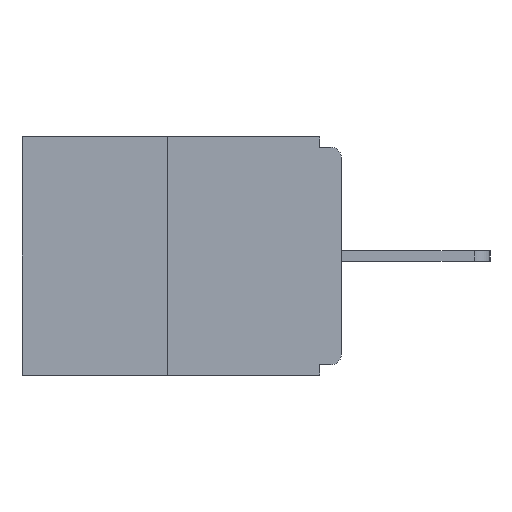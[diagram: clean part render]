
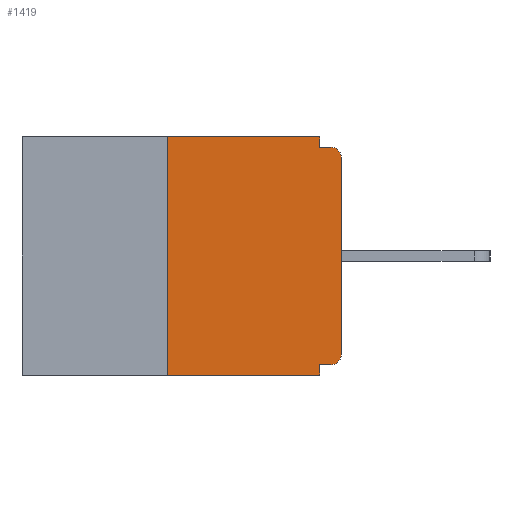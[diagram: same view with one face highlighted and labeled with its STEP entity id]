
A CAD part, left-side view. The second image highlights one B-rep face of the part: STEP entity #1419.
In plain terms, the highlighted planar face has unit normal (-1, 0, 0).
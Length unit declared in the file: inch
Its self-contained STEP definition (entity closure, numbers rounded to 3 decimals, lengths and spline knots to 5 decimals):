
#218 = VERTEX_POINT ( 'NONE', #4990 ) ;
#247 = VERTEX_POINT ( 'NONE', #21873 ) ;
#273 = LINE ( 'NONE', #2394, #9201 ) ;
#301 = CIRCLE ( 'NONE', #13572, 0.015 ) ;
#479 = LINE ( 'NONE', #7695, #22213 ) ;
#814 = DIRECTION ( 'NONE',  ( 0., 0., 1. ) ) ;
#1419 = ADVANCED_FACE ( 'NONE', ( #20451 ), #12638, .F. ) ;
#1489 = DIRECTION ( 'NONE',  ( 1., 0., 0. ) ) ;
#1607 = VECTOR ( 'NONE', #2393, 39.37008 ) ;
#1997 = CARTESIAN_POINT ( 'NONE',  ( 0., 0.031, -0.343 ) ) ;
#2081 = VECTOR ( 'NONE', #15148, 39.37008 ) ;
#2185 = LINE ( 'NONE', #17173, #2081 ) ;
#2393 = DIRECTION ( 'NONE',  ( 0., 0., -1. ) ) ;
#2394 = CARTESIAN_POINT ( 'NONE',  ( 0., 0., -0.015 ) ) ;
#2849 = EDGE_CURVE ( 'NONE', #15217, #17095, #2185, .T. ) ;
#3319 = EDGE_CURVE ( 'NONE', #11596, #247, #479, .T. ) ;
#4198 = ORIENTED_EDGE ( 'NONE', *, *, #2849, .F. ) ;
#4282 = LINE ( 'NONE', #9743, #1607 ) ;
#4823 = ORIENTED_EDGE ( 'NONE', *, *, #10709, .F. ) ;
#4830 = DIRECTION ( 'NONE',  ( 0., 0., -1. ) ) ;
#4950 = ORIENTED_EDGE ( 'NONE', *, *, #3319, .T. ) ;
#4990 = CARTESIAN_POINT ( 'NONE',  ( 0., 0.031, 0. ) ) ;
#5284 = EDGE_CURVE ( 'NONE', #11596, #22111, #11060, .T. ) ;
#5548 = LINE ( 'NONE', #1997, #19799 ) ;
#5707 = DIRECTION ( 'NONE',  ( 0., 0., 1. ) ) ;
#6445 = DIRECTION ( 'NONE',  ( 0., -1., 0. ) ) ;
#7033 = CARTESIAN_POINT ( 'NONE',  ( 0., 0.46, 0. ) ) ;
#7054 = ORIENTED_EDGE ( 'NONE', *, *, #21205, .F. ) ;
#7293 = CARTESIAN_POINT ( 'NONE',  ( 0., 0.015, -0.313 ) ) ;
#7461 = ORIENTED_EDGE ( 'NONE', *, *, #16400, .T. ) ;
#7664 = DIRECTION ( 'NONE',  ( 0., 0., -1. ) ) ;
#7695 = CARTESIAN_POINT ( 'NONE',  ( 0., 0.46, -0.343 ) ) ;
#9201 = VECTOR ( 'NONE', #16448, 39.37008 ) ;
#9293 = VECTOR ( 'NONE', #814, 39.37008 ) ;
#9549 = DIRECTION ( 'NONE',  ( -1., 0., 0. ) ) ;
#9743 = CARTESIAN_POINT ( 'NONE',  ( 0., 0.031, 0. ) ) ;
#9763 = VERTEX_POINT ( 'NONE', #18137 ) ;
#9778 = CARTESIAN_POINT ( 'NONE',  ( 0., 0., -0.313 ) ) ;
#10496 = VECTOR ( 'NONE', #5707, 39.37008 ) ;
#10709 = EDGE_CURVE ( 'NONE', #17095, #247, #5548, .T. ) ;
#11039 = CARTESIAN_POINT ( 'NONE',  ( 0., 0.031, -0.328 ) ) ;
#11060 = LINE ( 'NONE', #11299, #10496 ) ;
#11299 = CARTESIAN_POINT ( 'NONE',  ( 0., 0.25, 0. ) ) ;
#11584 = EDGE_CURVE ( 'NONE', #22111, #218, #15273, .T. ) ;
#11596 = VERTEX_POINT ( 'NONE', #22624 ) ;
#11966 = ORIENTED_EDGE ( 'NONE', *, *, #12019, .F. ) ;
#11976 = ORIENTED_EDGE ( 'NONE', *, *, #5284, .F. ) ;
#12019 = EDGE_CURVE ( 'NONE', #218, #16827, #4282, .T. ) ;
#12638 = PLANE ( 'NONE',  #12646 ) ;
#12646 = AXIS2_PLACEMENT_3D ( 'NONE', #7033, #1489, #14985 ) ;
#13403 = LINE ( 'NONE', #17122, #9293 ) ;
#13423 = CARTESIAN_POINT ( 'NONE',  ( 0., 0.031, -0.015 ) ) ;
#13515 = DIRECTION ( 'NONE',  ( -1., 0., 0. ) ) ;
#13572 = AXIS2_PLACEMENT_3D ( 'NONE', #18893, #13515, #4830 ) ;
#14664 = VERTEX_POINT ( 'NONE', #18934 ) ;
#14706 = DIRECTION ( 'NONE',  ( 0., 0., -1. ) ) ;
#14985 = DIRECTION ( 'NONE',  ( 0., 0., -1. ) ) ;
#14991 = DIRECTION ( 'NONE',  ( 0., -1., 0. ) ) ;
#15148 = DIRECTION ( 'NONE',  ( 0., 1., 0. ) ) ;
#15217 = VERTEX_POINT ( 'NONE', #18598 ) ;
#15273 = LINE ( 'NONE', #22747, #17948 ) ;
#15507 = AXIS2_PLACEMENT_3D ( 'NONE', #7293, #9549, #14706 ) ;
#16074 = EDGE_CURVE ( 'NONE', #9763, #14664, #301, .T. ) ;
#16400 = EDGE_CURVE ( 'NONE', #15217, #22818, #23084, .T. ) ;
#16448 = DIRECTION ( 'NONE',  ( 0., -1., 0. ) ) ;
#16827 = VERTEX_POINT ( 'NONE', #13423 ) ;
#17095 = VERTEX_POINT ( 'NONE', #11039 ) ;
#17122 = CARTESIAN_POINT ( 'NONE',  ( 0., 0., 0. ) ) ;
#17173 = CARTESIAN_POINT ( 'NONE',  ( 0., 0., -0.328 ) ) ;
#17948 = VECTOR ( 'NONE', #6445, 39.37008 ) ;
#18137 = CARTESIAN_POINT ( 'NONE',  ( 0., 0., -0.03 ) ) ;
#18158 = EDGE_LOOP ( 'NONE', ( #22549, #11976, #4950, #4823, #4198, #7461, #19357, #22069, #7054, #11966 ) ) ;
#18598 = CARTESIAN_POINT ( 'NONE',  ( 0., 0.015, -0.328 ) ) ;
#18893 = CARTESIAN_POINT ( 'NONE',  ( 0., 0.015, -0.03 ) ) ;
#18934 = CARTESIAN_POINT ( 'NONE',  ( 0., 0.015, -0.015 ) ) ;
#19357 = ORIENTED_EDGE ( 'NONE', *, *, #23196, .T. ) ;
#19440 = CARTESIAN_POINT ( 'NONE',  ( 0., 0.25, 0. ) ) ;
#19799 = VECTOR ( 'NONE', #7664, 39.37008 ) ;
#20451 = FACE_OUTER_BOUND ( 'NONE', #18158, .T. ) ;
#21205 = EDGE_CURVE ( 'NONE', #16827, #14664, #273, .T. ) ;
#21873 = CARTESIAN_POINT ( 'NONE',  ( 0., 0.031, -0.343 ) ) ;
#22069 = ORIENTED_EDGE ( 'NONE', *, *, #16074, .T. ) ;
#22111 = VERTEX_POINT ( 'NONE', #19440 ) ;
#22213 = VECTOR ( 'NONE', #14991, 39.37008 ) ;
#22549 = ORIENTED_EDGE ( 'NONE', *, *, #11584, .F. ) ;
#22624 = CARTESIAN_POINT ( 'NONE',  ( 0., 0.25, -0.343 ) ) ;
#22747 = CARTESIAN_POINT ( 'NONE',  ( 0., 0.46, 0. ) ) ;
#22818 = VERTEX_POINT ( 'NONE', #9778 ) ;
#23084 = CIRCLE ( 'NONE', #15507, 0.015 ) ;
#23196 = EDGE_CURVE ( 'NONE', #22818, #9763, #13403, .T. ) ;
